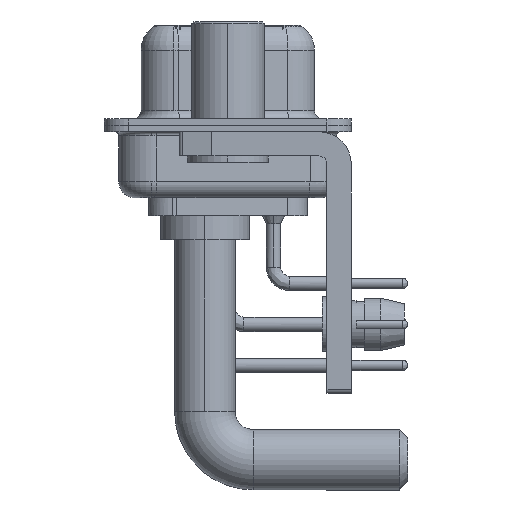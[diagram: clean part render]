
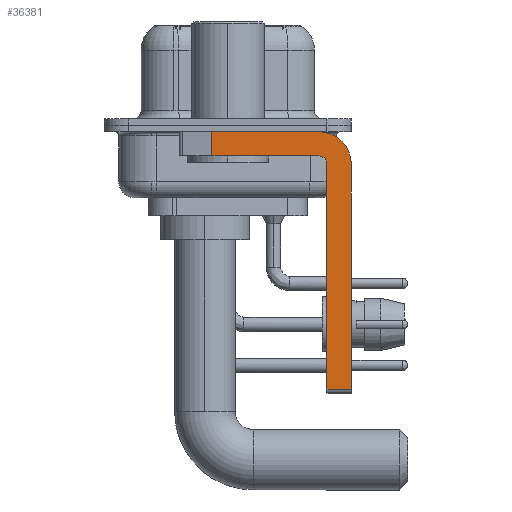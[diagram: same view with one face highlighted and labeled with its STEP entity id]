
A CAD part, left-side view. The second image highlights one B-rep face of the part: STEP entity #36381.
In plain terms, the highlighted planar face has unit normal (-1, 0, 0).
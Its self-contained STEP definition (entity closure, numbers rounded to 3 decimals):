
#749 = ORIENTED_EDGE ( 'NONE', *, *, #36599, .F. ) ;
#763 = CARTESIAN_POINT ( 'NONE',  ( -2.9, -7.65, -2.4 ) ) ;
#994 = DIRECTION ( 'NONE',  ( 0., -1., 0. ) ) ;
#1219 = CARTESIAN_POINT ( 'NONE',  ( -2.9, -7.65, -16.35 ) ) ;
#1838 = VERTEX_POINT ( 'NONE', #17440 ) ;
#1937 = DIRECTION ( 'NONE',  ( 0., 0., -1. ) ) ;
#1989 = EDGE_CURVE ( 'NONE', #25869, #1838, #21791, .T. ) ;
#2365 = VERTEX_POINT ( 'NONE', #1219 ) ;
#2768 = CARTESIAN_POINT ( 'NONE',  ( -2.9, -5.65, -2.4 ) ) ;
#2889 = DIRECTION ( 'NONE',  ( 0., 0., -1. ) ) ;
#3984 = VERTEX_POINT ( 'NONE', #17901 ) ;
#4200 = VERTEX_POINT ( 'NONE', #14420 ) ;
#4358 = AXIS2_PLACEMENT_3D ( 'NONE', #31044, #34422, #20549 ) ;
#5251 = CIRCLE ( 'NONE', #34348, 2. ) ;
#5329 = VECTOR ( 'NONE', #28230, 1000. ) ;
#5441 = VECTOR ( 'NONE', #29549, 1000. ) ;
#5465 = VECTOR ( 'NONE', #1937, 1000. ) ;
#5929 = CARTESIAN_POINT ( 'NONE',  ( -2.9, -5.65, -2.4 ) ) ;
#6025 = VECTOR ( 'NONE', #32076, 1000. ) ;
#6627 = ORIENTED_EDGE ( 'NONE', *, *, #26580, .T. ) ;
#6827 = ORIENTED_EDGE ( 'NONE', *, *, #10469, .T. ) ;
#7247 = CARTESIAN_POINT ( 'NONE',  ( -2.9, 0.978, -1.9 ) ) ;
#7455 = LINE ( 'NONE', #7247, #5465 ) ;
#9231 = CARTESIAN_POINT ( 'NONE',  ( -2.9, 0.978, -0.4 ) ) ;
#9943 = CARTESIAN_POINT ( 'NONE',  ( -2.9, -5.65, -16.35 ) ) ;
#10469 = EDGE_CURVE ( 'NONE', #4200, #2365, #21355, .T. ) ;
#11774 = ORIENTED_EDGE ( 'NONE', *, *, #19441, .F. ) ;
#13624 = CARTESIAN_POINT ( 'NONE',  ( -2.9, 3., -0.4 ) ) ;
#14420 = CARTESIAN_POINT ( 'NONE',  ( -2.9, -6.15, -16.35 ) ) ;
#14561 = FACE_OUTER_BOUND ( 'NONE', #34816, .T. ) ;
#15155 = VERTEX_POINT ( 'NONE', #24834 ) ;
#15200 = LINE ( 'NONE', #23375, #6025 ) ;
#17101 = CARTESIAN_POINT ( 'NONE',  ( -2.9, 0.978, -1.9 ) ) ;
#17440 = CARTESIAN_POINT ( 'NONE',  ( -2.9, -5.65, -0.4 ) ) ;
#17901 = CARTESIAN_POINT ( 'NONE',  ( -2.9, -6.15, -2.4 ) ) ;
#19441 = EDGE_CURVE ( 'NONE', #1838, #20118, #5251, .T. ) ;
#19532 = CIRCLE ( 'NONE', #4358, 0.5 ) ;
#20118 = VERTEX_POINT ( 'NONE', #763 ) ;
#20549 = DIRECTION ( 'NONE',  ( 0., 0., 1. ) ) ;
#21355 = LINE ( 'NONE', #9943, #26813 ) ;
#21723 = VERTEX_POINT ( 'NONE', #17101 ) ;
#21791 = LINE ( 'NONE', #13624, #5329 ) ;
#22434 = AXIS2_PLACEMENT_3D ( 'NONE', #2768, #26497, #37302 ) ;
#23324 = EDGE_CURVE ( 'NONE', #4200, #3984, #24044, .T. ) ;
#23364 = ORIENTED_EDGE ( 'NONE', *, *, #29981, .F. ) ;
#23375 = CARTESIAN_POINT ( 'NONE',  ( -2.9, -5.65, -1.9 ) ) ;
#23603 = DIRECTION ( 'NONE',  ( 1., 0., 0. ) ) ;
#24044 = LINE ( 'NONE', #35251, #5441 ) ;
#24581 = CARTESIAN_POINT ( 'NONE',  ( -2.9, -7.65, -2.4 ) ) ;
#24834 = CARTESIAN_POINT ( 'NONE',  ( -2.9, -5.65, -1.9 ) ) ;
#25181 = ORIENTED_EDGE ( 'NONE', *, *, #1989, .F. ) ;
#25869 = VERTEX_POINT ( 'NONE', #9231 ) ;
#26497 = DIRECTION ( 'NONE',  ( 1., 0., 0. ) ) ;
#26580 = EDGE_CURVE ( 'NONE', #25869, #21723, #7455, .T. ) ;
#26813 = VECTOR ( 'NONE', #994, 1000. ) ;
#26888 = DIRECTION ( 'NONE',  ( 0., 0., -1. ) ) ;
#27247 = LINE ( 'NONE', #24581, #27870 ) ;
#27870 = VECTOR ( 'NONE', #26888, 1000. ) ;
#28230 = DIRECTION ( 'NONE',  ( 0., -1., 0. ) ) ;
#28647 = ORIENTED_EDGE ( 'NONE', *, *, #23324, .F. ) ;
#29549 = DIRECTION ( 'NONE',  ( 0., 0., 1. ) ) ;
#29901 = ORIENTED_EDGE ( 'NONE', *, *, #31880, .F. ) ;
#29981 = EDGE_CURVE ( 'NONE', #15155, #21723, #15200, .T. ) ;
#31044 = CARTESIAN_POINT ( 'NONE',  ( -2.9, -5.65, -2.4 ) ) ;
#31880 = EDGE_CURVE ( 'NONE', #3984, #15155, #19532, .T. ) ;
#32076 = DIRECTION ( 'NONE',  ( 0., 1., 0. ) ) ;
#34348 = AXIS2_PLACEMENT_3D ( 'NONE', #5929, #23603, #2889 ) ;
#34422 = DIRECTION ( 'NONE',  ( -1., 0., 0. ) ) ;
#34473 = PLANE ( 'NONE',  #22434 ) ;
#34816 = EDGE_LOOP ( 'NONE', ( #25181, #6627, #23364, #29901, #28647, #6827, #749, #11774 ) ) ;
#35251 = CARTESIAN_POINT ( 'NONE',  ( -2.9, -6.15, -16.6 ) ) ;
#36381 = ADVANCED_FACE ( 'NONE', ( #14561 ), #34473, .F. ) ;
#36599 = EDGE_CURVE ( 'NONE', #20118, #2365, #27247, .T. ) ;
#37302 = DIRECTION ( 'NONE',  ( 0., 0., -1. ) ) ;
